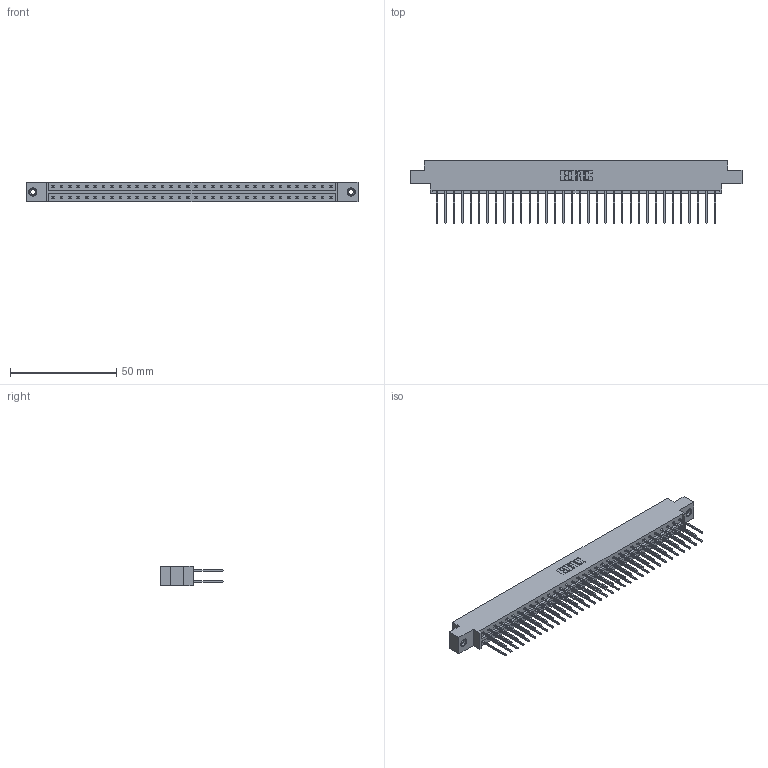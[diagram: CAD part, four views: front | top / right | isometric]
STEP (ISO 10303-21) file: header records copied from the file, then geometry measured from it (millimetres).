
FILE_DESCRIPTION (( 'STEP AP203' ), '1' );
FILE_NAME ('833-068-540-808.STEP', '2020-06-05T10:39:00', ( '' ), ( '' ), 'SwSTEP 2.0', 'SolidWorks 2020', '' );
FILE_SCHEMA (( 'CONFIG_CONTROL_DESIGN' ));
Length unit declared in the file: inch
Products named in the file (4): 833-068-540-808; 345-292-001_345-293-140; 345-250-001_345-250-003-102; 833 Part_Offset - .156 Dia - TI
Assembly tree (71 placements, depth 2):
  833-068-540-808
    833 Part_Offset - .156 Dia - TI
    345-292-001_345-293-140  x68
    345-250-001_345-250-003-102  x2
Bounding box: 156.26 x 29.47 x 9.4 mm (x, y, z)
Volume: 15902 mm3; surface area: 20222.2 mm2
Topology: 71 solids, 71 shells, 3714 faces, 10999 edges, 7234 vertices
Faces by surface type: plane 2554, cylinder 1144, cone 12, torus 4
Entity records: 24244 total; most frequent: CARTESIAN_POINT 4013, ORIENTED_EDGE 3942, DIRECTION 3473, EDGE_CURVE 1971, LINE 1823, VECTOR 1823, VERTEX_POINT 1308, AXIS2_PLACEMENT_3D 825
